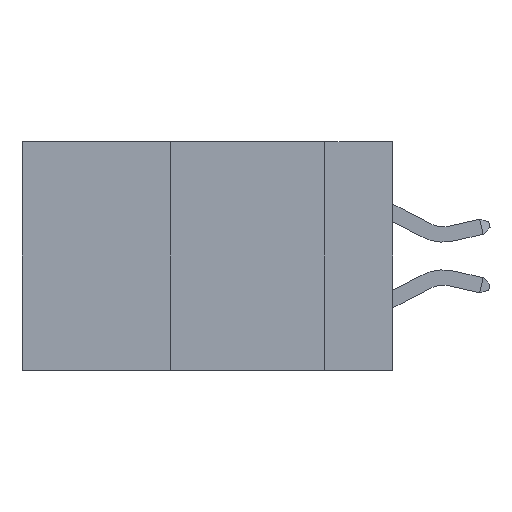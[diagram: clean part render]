
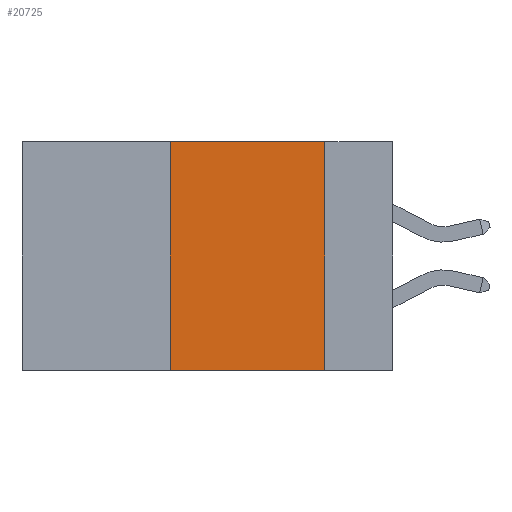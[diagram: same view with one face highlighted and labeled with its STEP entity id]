
A CAD part, left-side view. The second image highlights one B-rep face of the part: STEP entity #20725.
In plain terms, the highlighted planar face has unit normal (-1, 0, 0).
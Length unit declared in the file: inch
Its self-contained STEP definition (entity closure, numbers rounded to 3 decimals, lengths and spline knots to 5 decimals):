
#1103 = AXIS2_PLACEMENT_3D ( 'NONE', #8590, #18723, #13887 ) ;
#1851 = CARTESIAN_POINT ( 'NONE',  ( 0., 0.11, 0. ) ) ;
#2082 = VECTOR ( 'NONE', #6484, 39.37008 ) ;
#3026 = ORIENTED_EDGE ( 'NONE', *, *, #20153, .F. ) ;
#3689 = EDGE_CURVE ( 'NONE', #15672, #7574, #12709, .T. ) ;
#4204 = ORIENTED_EDGE ( 'NONE', *, *, #8180, .F. ) ;
#4950 = VERTEX_POINT ( 'NONE', #5453 ) ;
#5025 = FACE_OUTER_BOUND ( 'NONE', #9281, .T. ) ;
#5453 = CARTESIAN_POINT ( 'NONE',  ( 0., 0.11, 0. ) ) ;
#6484 = DIRECTION ( 'NONE',  ( 0., 0., 1. ) ) ;
#7574 = VERTEX_POINT ( 'NONE', #15248 ) ;
#8180 = EDGE_CURVE ( 'NONE', #4950, #7574, #15658, .T. ) ;
#8590 = CARTESIAN_POINT ( 'NONE',  ( 0., 0.6, 0. ) ) ;
#8907 = EDGE_CURVE ( 'NONE', #15672, #22590, #20306, .T. ) ;
#9281 = EDGE_LOOP ( 'NONE', ( #4204, #3026, #18484, #10143 ) ) ;
#10143 = ORIENTED_EDGE ( 'NONE', *, *, #3689, .T. ) ;
#10716 = DIRECTION ( 'NONE',  ( 0., -1., 0. ) ) ;
#11588 = VECTOR ( 'NONE', #17713, 39.37008 ) ;
#12709 = LINE ( 'NONE', #19612, #13814 ) ;
#12900 = CARTESIAN_POINT ( 'NONE',  ( 0., 0.6, 0. ) ) ;
#13646 = CARTESIAN_POINT ( 'NONE',  ( 0., 0.36, -0.37 ) ) ;
#13814 = VECTOR ( 'NONE', #16154, 39.37008 ) ;
#13887 = DIRECTION ( 'NONE',  ( 0., 0., -1. ) ) ;
#15248 = CARTESIAN_POINT ( 'NONE',  ( 0., 0.11, -0.37 ) ) ;
#15658 = LINE ( 'NONE', #1851, #11588 ) ;
#15672 = VERTEX_POINT ( 'NONE', #13646 ) ;
#16154 = DIRECTION ( 'NONE',  ( 0., -1., 0. ) ) ;
#16346 = LINE ( 'NONE', #12900, #20547 ) ;
#17100 = CARTESIAN_POINT ( 'NONE',  ( 0., 0.36, 0. ) ) ;
#17124 = PLANE ( 'NONE',  #1103 ) ;
#17713 = DIRECTION ( 'NONE',  ( 0., 0., -1. ) ) ;
#18484 = ORIENTED_EDGE ( 'NONE', *, *, #8907, .F. ) ;
#18723 = DIRECTION ( 'NONE',  ( 1., 0., 0. ) ) ;
#18933 = CARTESIAN_POINT ( 'NONE',  ( 0., 0.36, 0. ) ) ;
#19612 = CARTESIAN_POINT ( 'NONE',  ( 0., 0.6, -0.37 ) ) ;
#20153 = EDGE_CURVE ( 'NONE', #22590, #4950, #16346, .T. ) ;
#20306 = LINE ( 'NONE', #18933, #2082 ) ;
#20547 = VECTOR ( 'NONE', #10716, 39.37008 ) ;
#20725 = ADVANCED_FACE ( 'NONE', ( #5025 ), #17124, .F. ) ;
#22590 = VERTEX_POINT ( 'NONE', #17100 ) ;
